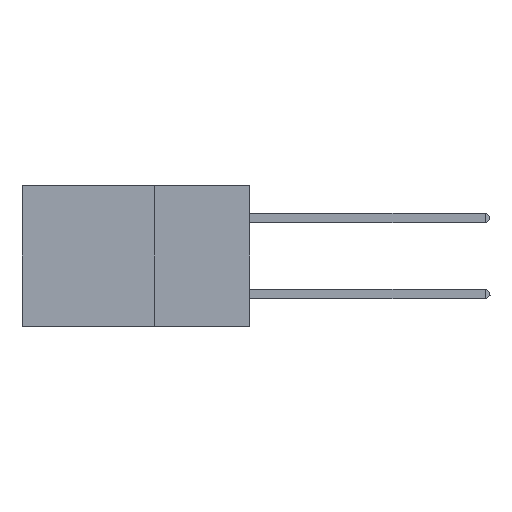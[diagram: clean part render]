
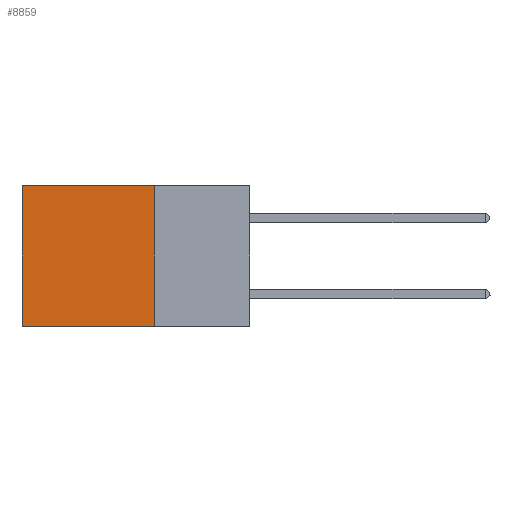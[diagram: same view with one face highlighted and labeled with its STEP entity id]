
A CAD part, left-side view. The second image highlights one B-rep face of the part: STEP entity #8859.
In plain terms, the highlighted planar face has unit normal (-1, 0, 0).
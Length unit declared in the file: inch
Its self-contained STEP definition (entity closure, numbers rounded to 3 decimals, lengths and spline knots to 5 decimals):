
#246 = EDGE_CURVE ( 'NONE', #9918, #2578, #13882, .T. ) ;
#675 = EDGE_CURVE ( 'NONE', #9918, #13975, #5089, .T. ) ;
#1014 = PLANE ( 'NONE',  #15228 ) ;
#1024 = DIRECTION ( 'NONE',  ( 0., 0., -1. ) ) ;
#2347 = VECTOR ( 'NONE', #1024, 39.37008 ) ;
#2578 = VERTEX_POINT ( 'NONE', #10194 ) ;
#2816 = EDGE_LOOP ( 'NONE', ( #9256, #6751, #15534, #12759 ) ) ;
#3531 = EDGE_CURVE ( 'NONE', #13975, #5849, #9087, .T. ) ;
#3857 = CARTESIAN_POINT ( 'NONE',  ( 0.2875, 0.6, -0.37 ) ) ;
#4541 = FACE_OUTER_BOUND ( 'NONE', #2816, .T. ) ;
#4723 = DIRECTION ( 'NONE',  ( 0., 1., 0. ) ) ;
#5052 = DIRECTION ( 'NONE',  ( 1., 0., 0. ) ) ;
#5089 = LINE ( 'NONE', #8569, #11658 ) ;
#5849 = VERTEX_POINT ( 'NONE', #3857 ) ;
#5925 = DIRECTION ( 'NONE',  ( 0., 1., 0. ) ) ;
#6751 = ORIENTED_EDGE ( 'NONE', *, *, #3531, .F. ) ;
#6938 = EDGE_CURVE ( 'NONE', #2578, #5849, #8581, .T. ) ;
#7409 = CARTESIAN_POINT ( 'NONE',  ( 0.2875, 0.6, 0. ) ) ;
#8569 = CARTESIAN_POINT ( 'NONE',  ( 0.2875, 0.25, 0. ) ) ;
#8581 = LINE ( 'NONE', #7409, #2347 ) ;
#8859 = ADVANCED_FACE ( 'NONE', ( #4541 ), #1014, .F. ) ;
#9087 = LINE ( 'NONE', #11093, #15908 ) ;
#9256 = ORIENTED_EDGE ( 'NONE', *, *, #6938, .T. ) ;
#9918 = VERTEX_POINT ( 'NONE', #16539 ) ;
#10194 = CARTESIAN_POINT ( 'NONE',  ( 0.2875, 0.6, 0. ) ) ;
#10473 = VECTOR ( 'NONE', #5925, 39.37008 ) ;
#11093 = CARTESIAN_POINT ( 'NONE',  ( 0.2875, 0.25, -0.37 ) ) ;
#11658 = VECTOR ( 'NONE', #15098, 39.37008 ) ;
#12759 = ORIENTED_EDGE ( 'NONE', *, *, #246, .T. ) ;
#13815 = DIRECTION ( 'NONE',  ( 0., 0., -1. ) ) ;
#13882 = LINE ( 'NONE', #13939, #10473 ) ;
#13883 = CARTESIAN_POINT ( 'NONE',  ( 0.2875, 0.25, -0.37 ) ) ;
#13939 = CARTESIAN_POINT ( 'NONE',  ( 0.2875, 0.25, 0. ) ) ;
#13975 = VERTEX_POINT ( 'NONE', #13883 ) ;
#14843 = CARTESIAN_POINT ( 'NONE',  ( 0.2875, 0.25, 0. ) ) ;
#15098 = DIRECTION ( 'NONE',  ( 0., 0., -1. ) ) ;
#15228 = AXIS2_PLACEMENT_3D ( 'NONE', #14843, #5052, #13815 ) ;
#15534 = ORIENTED_EDGE ( 'NONE', *, *, #675, .F. ) ;
#15908 = VECTOR ( 'NONE', #4723, 39.37008 ) ;
#16539 = CARTESIAN_POINT ( 'NONE',  ( 0.2875, 0.25, 0. ) ) ;
